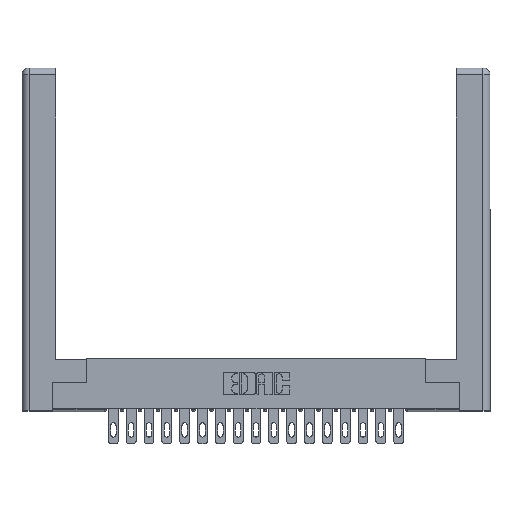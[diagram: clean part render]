
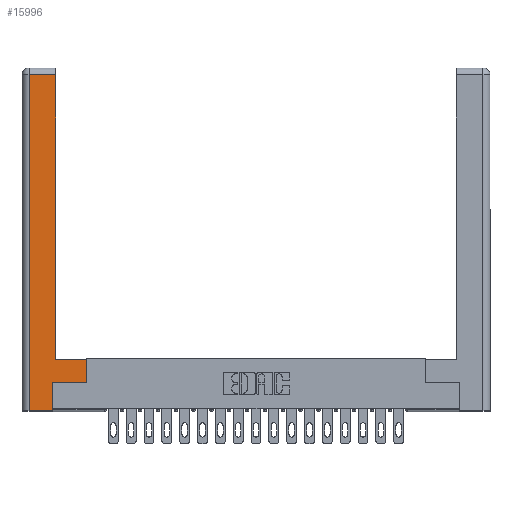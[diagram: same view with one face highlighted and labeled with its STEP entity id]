
A CAD part, top view. The second image highlights one B-rep face of the part: STEP entity #15996.
In plain terms, the highlighted planar face has unit normal (0, 0, 1).
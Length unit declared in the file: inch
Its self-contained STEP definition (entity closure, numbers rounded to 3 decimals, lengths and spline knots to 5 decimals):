
#383 = EDGE_LOOP ( 'NONE', ( #3499, #13979, #2585, #2811, #12652, #15142, #5799, #18724 ) ) ;
#602 = VECTOR ( 'NONE', #3125, 39.37008 ) ;
#731 = EDGE_CURVE ( 'NONE', #1997, #11975, #4651, .T. ) ;
#757 = CARTESIAN_POINT ( 'NONE',  ( 0.265, 0., 0. ) ) ;
#904 = CARTESIAN_POINT ( 'NONE',  ( 0.265, 0.245, 0. ) ) ;
#988 = DIRECTION ( 'NONE',  ( 1., 0., 0. ) ) ;
#1976 = LINE ( 'NONE', #6742, #16890 ) ;
#1997 = VERTEX_POINT ( 'NONE', #11069 ) ;
#2585 = ORIENTED_EDGE ( 'NONE', *, *, #17502, .T. ) ;
#2732 = DIRECTION ( 'NONE',  ( 0., 0., -1. ) ) ;
#2811 = ORIENTED_EDGE ( 'NONE', *, *, #731, .T. ) ;
#3125 = DIRECTION ( 'NONE',  ( 0., -1., 0. ) ) ;
#3275 = EDGE_CURVE ( 'NONE', #11975, #20633, #10762, .T. ) ;
#3499 = ORIENTED_EDGE ( 'NONE', *, *, #4657, .T. ) ;
#3508 = CARTESIAN_POINT ( 'NONE',  ( 0.295, 2.94, 0. ) ) ;
#4117 = CARTESIAN_POINT ( 'NONE',  ( 0.565, 0.245, 0. ) ) ;
#4397 = VECTOR ( 'NONE', #14425, 39.37008 ) ;
#4437 = DIRECTION ( 'NONE',  ( 0., 1., 0. ) ) ;
#4651 = LINE ( 'NONE', #6311, #15894 ) ;
#4657 = EDGE_CURVE ( 'NONE', #14409, #5044, #1976, .T. ) ;
#4700 = CARTESIAN_POINT ( 'NONE',  ( 0.0615, 2.94, 0. ) ) ;
#5044 = VERTEX_POINT ( 'NONE', #3508 ) ;
#5117 = CARTESIAN_POINT ( 'NONE',  ( 0.565, 0.45, 0. ) ) ;
#5676 = LINE ( 'NONE', #4117, #5748 ) ;
#5748 = VECTOR ( 'NONE', #8789, 39.37008 ) ;
#5799 = ORIENTED_EDGE ( 'NONE', *, *, #13913, .T. ) ;
#5875 = CARTESIAN_POINT ( 'NONE',  ( 0.565, 0.45, 0. ) ) ;
#6276 = DIRECTION ( 'NONE',  ( -1., 0., 0. ) ) ;
#6311 = CARTESIAN_POINT ( 'NONE',  ( 0.265, 0., 0. ) ) ;
#6330 = LINE ( 'NONE', #5875, #13269 ) ;
#6363 = EDGE_CURVE ( 'NONE', #5044, #17041, #8282, .T. ) ;
#6722 = DIRECTION ( 'NONE',  ( -1., 0., 0. ) ) ;
#6742 = CARTESIAN_POINT ( 'NONE',  ( 0.295, 3., 0. ) ) ;
#7479 = VERTEX_POINT ( 'NONE', #18830 ) ;
#8282 = LINE ( 'NONE', #15032, #14753 ) ;
#8789 = DIRECTION ( 'NONE',  ( 1., 0., 0. ) ) ;
#9495 = FACE_OUTER_BOUND ( 'NONE', #383, .T. ) ;
#9665 = CARTESIAN_POINT ( 'NONE',  ( 0.0615, 0., 0. ) ) ;
#10109 = VERTEX_POINT ( 'NONE', #5117 ) ;
#10762 = LINE ( 'NONE', #904, #4397 ) ;
#11069 = CARTESIAN_POINT ( 'NONE',  ( 0.0615, 0., 0. ) ) ;
#11219 = AXIS2_PLACEMENT_3D ( 'NONE', #17892, #2732, #6276 ) ;
#11523 = EDGE_CURVE ( 'NONE', #20633, #7479, #5676, .T. ) ;
#11975 = VERTEX_POINT ( 'NONE', #757 ) ;
#12038 = CARTESIAN_POINT ( 'NONE',  ( 0.295, 0.45, 0. ) ) ;
#12652 = ORIENTED_EDGE ( 'NONE', *, *, #3275, .T. ) ;
#13269 = VECTOR ( 'NONE', #4437, 39.37008 ) ;
#13372 = DIRECTION ( 'NONE',  ( -1., 0., 0. ) ) ;
#13913 = EDGE_CURVE ( 'NONE', #7479, #10109, #6330, .T. ) ;
#13979 = ORIENTED_EDGE ( 'NONE', *, *, #6363, .T. ) ;
#14409 = VERTEX_POINT ( 'NONE', #21774 ) ;
#14425 = DIRECTION ( 'NONE',  ( 0., 1., 0. ) ) ;
#14753 = VECTOR ( 'NONE', #13372, 39.37008 ) ;
#15032 = CARTESIAN_POINT ( 'NONE',  ( 0.0615, 2.94, 0. ) ) ;
#15033 = LINE ( 'NONE', #12038, #19394 ) ;
#15142 = ORIENTED_EDGE ( 'NONE', *, *, #11523, .T. ) ;
#15894 = VECTOR ( 'NONE', #988, 39.37008 ) ;
#15996 = ADVANCED_FACE ( 'NONE', ( #9495 ), #19337, .F. ) ;
#16890 = VECTOR ( 'NONE', #18798, 39.37008 ) ;
#17041 = VERTEX_POINT ( 'NONE', #4700 ) ;
#17502 = EDGE_CURVE ( 'NONE', #17041, #1997, #21524, .T. ) ;
#17892 = CARTESIAN_POINT ( 'NONE',  ( 0., 0., 0. ) ) ;
#18339 = CARTESIAN_POINT ( 'NONE',  ( 0.265, 0.245, 0. ) ) ;
#18501 = EDGE_CURVE ( 'NONE', #10109, #14409, #15033, .T. ) ;
#18724 = ORIENTED_EDGE ( 'NONE', *, *, #18501, .T. ) ;
#18798 = DIRECTION ( 'NONE',  ( 0., 1., 0. ) ) ;
#18830 = CARTESIAN_POINT ( 'NONE',  ( 0.565, 0.245, 0. ) ) ;
#19337 = PLANE ( 'NONE',  #11219 ) ;
#19394 = VECTOR ( 'NONE', #6722, 39.37008 ) ;
#20633 = VERTEX_POINT ( 'NONE', #18339 ) ;
#21524 = LINE ( 'NONE', #9665, #602 ) ;
#21774 = CARTESIAN_POINT ( 'NONE',  ( 0.295, 0.45, 0. ) ) ;
